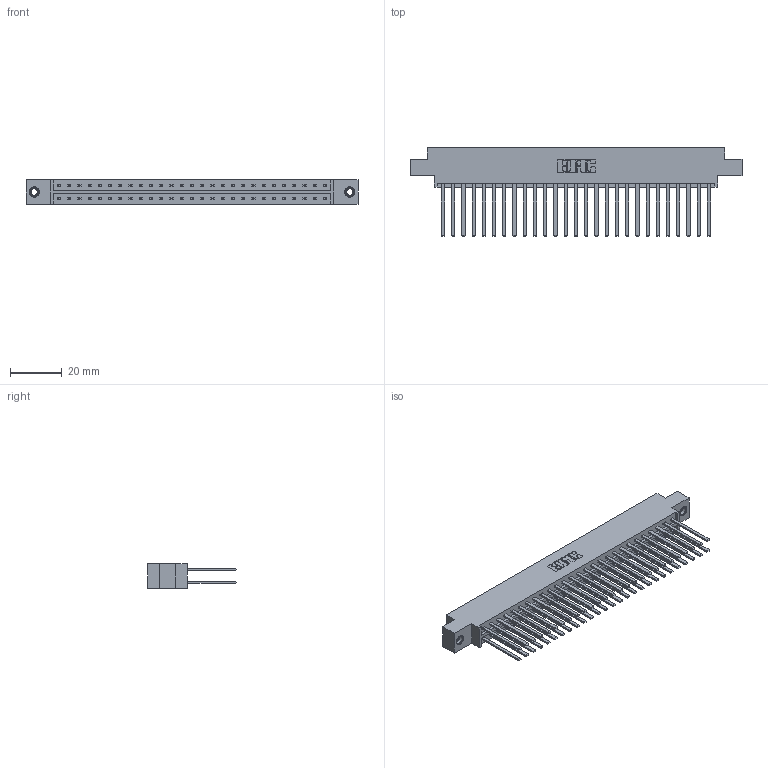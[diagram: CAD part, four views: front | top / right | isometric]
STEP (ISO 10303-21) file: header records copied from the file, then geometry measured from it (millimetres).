
FILE_DESCRIPTION (( 'STEP AP203' ), '1' );
FILE_NAME ('833-054-544-807.STEP', '2020-06-04T21:19:18', ( '' ), ( '' ), 'SwSTEP 2.0', 'SolidWorks 2020', '' );
FILE_SCHEMA (( 'CONFIG_CONTROL_DESIGN' ));
Length unit declared in the file: inch
Products named in the file (4): 345-250-001_345-250-005-103; 345-292-001_345-293-144; 833-054-544-807; 833 Part_Offset - .156 Dia - TI
Assembly tree (57 placements, depth 2):
  833-054-544-807
    833 Part_Offset - .156 Dia - TI
    345-292-001_345-293-144  x54
    345-250-001_345-250-005-103  x2
Bounding box: 128.52 x 34.3 x 9.4 mm (x, y, z)
Volume: 13497 mm3; surface area: 18487.8 mm2
Topology: 57 solids, 57 shells, 2662 faces, 7857 edges, 5158 vertices
Faces by surface type: plane 1834, cylinder 812, cone 12, torus 4
Entity records: 20444 total; most frequent: CARTESIAN_POINT 3389, ORIENTED_EDGE 3318, DIRECTION 2949, EDGE_CURVE 1659, VECTOR 1515, LINE 1515, VERTEX_POINT 1100, AXIS2_PLACEMENT_3D 717
